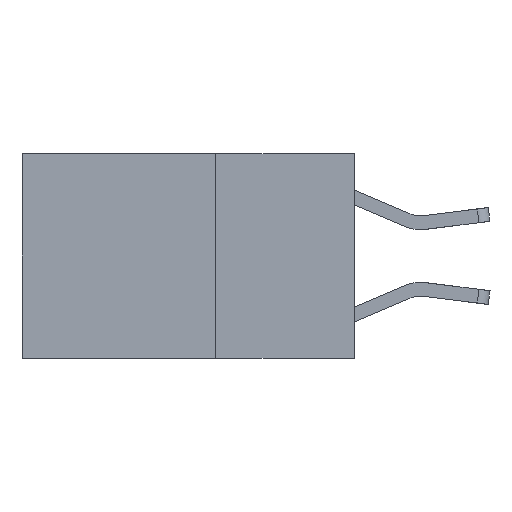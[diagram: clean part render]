
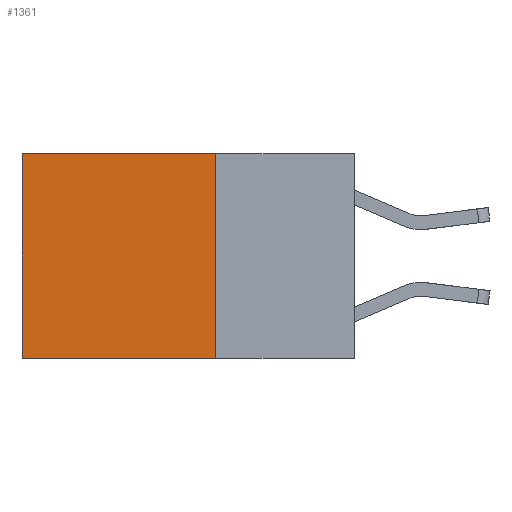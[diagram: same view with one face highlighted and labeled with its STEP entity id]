
A CAD part, left-side view. The second image highlights one B-rep face of the part: STEP entity #1361.
In plain terms, the highlighted planar face has unit normal (-1, 0, 0).
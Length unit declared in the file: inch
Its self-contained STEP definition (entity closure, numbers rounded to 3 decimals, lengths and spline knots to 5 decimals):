
#251 = DIRECTION ( 'NONE',  ( 0., 0., -1. ) ) ;
#297 = CARTESIAN_POINT ( 'NONE',  ( 0.2625, 0.6, 0. ) ) ;
#420 = VECTOR ( 'NONE', #2250, 39.37008 ) ;
#804 = CARTESIAN_POINT ( 'NONE',  ( 0.2625, 0.25, 0. ) ) ;
#826 = CARTESIAN_POINT ( 'NONE',  ( 0.2625, 0.25, 0. ) ) ;
#947 = EDGE_CURVE ( 'NONE', #1847, #4460, #4395, .T. ) ;
#1187 = ORIENTED_EDGE ( 'NONE', *, *, #947, .F. ) ;
#1345 = ORIENTED_EDGE ( 'NONE', *, *, #6308, .F. ) ;
#1361 = ADVANCED_FACE ( 'NONE', ( #1393 ), #4234, .F. ) ;
#1393 = FACE_OUTER_BOUND ( 'NONE', #1443, .T. ) ;
#1443 = EDGE_LOOP ( 'NONE', ( #6559, #1187, #1345, #6815 ) ) ;
#1639 = LINE ( 'NONE', #297, #420 ) ;
#1832 = VECTOR ( 'NONE', #251, 39.37008 ) ;
#1847 = VERTEX_POINT ( 'NONE', #3002 ) ;
#2154 = VERTEX_POINT ( 'NONE', #6980 ) ;
#2250 = DIRECTION ( 'NONE',  ( 0., 0., -1. ) ) ;
#2313 = VERTEX_POINT ( 'NONE', #8576 ) ;
#2495 = CARTESIAN_POINT ( 'NONE',  ( 0.2625, 0.25, -0.37 ) ) ;
#3002 = CARTESIAN_POINT ( 'NONE',  ( 0.2625, 0.25, -0.37 ) ) ;
#3505 = LINE ( 'NONE', #8257, #1832 ) ;
#3547 = EDGE_CURVE ( 'NONE', #2154, #2313, #4026, .T. ) ;
#3944 = CARTESIAN_POINT ( 'NONE',  ( 0.2625, 0.6, -0.37 ) ) ;
#4026 = LINE ( 'NONE', #804, #5130 ) ;
#4234 = PLANE ( 'NONE',  #4852 ) ;
#4395 = LINE ( 'NONE', #2495, #7353 ) ;
#4460 = VERTEX_POINT ( 'NONE', #3944 ) ;
#4585 = EDGE_CURVE ( 'NONE', #2313, #4460, #1639, .T. ) ;
#4852 = AXIS2_PLACEMENT_3D ( 'NONE', #826, #6906, #6723 ) ;
#5130 = VECTOR ( 'NONE', #7992, 39.37008 ) ;
#6308 = EDGE_CURVE ( 'NONE', #2154, #1847, #3505, .T. ) ;
#6559 = ORIENTED_EDGE ( 'NONE', *, *, #4585, .T. ) ;
#6723 = DIRECTION ( 'NONE',  ( 0., 0., -1. ) ) ;
#6815 = ORIENTED_EDGE ( 'NONE', *, *, #3547, .T. ) ;
#6906 = DIRECTION ( 'NONE',  ( 1., 0., 0. ) ) ;
#6980 = CARTESIAN_POINT ( 'NONE',  ( 0.2625, 0.25, 0. ) ) ;
#7353 = VECTOR ( 'NONE', #8444, 39.37008 ) ;
#7992 = DIRECTION ( 'NONE',  ( 0., 1., 0. ) ) ;
#8257 = CARTESIAN_POINT ( 'NONE',  ( 0.2625, 0.25, 0. ) ) ;
#8444 = DIRECTION ( 'NONE',  ( 0., 1., 0. ) ) ;
#8576 = CARTESIAN_POINT ( 'NONE',  ( 0.2625, 0.6, 0. ) ) ;
